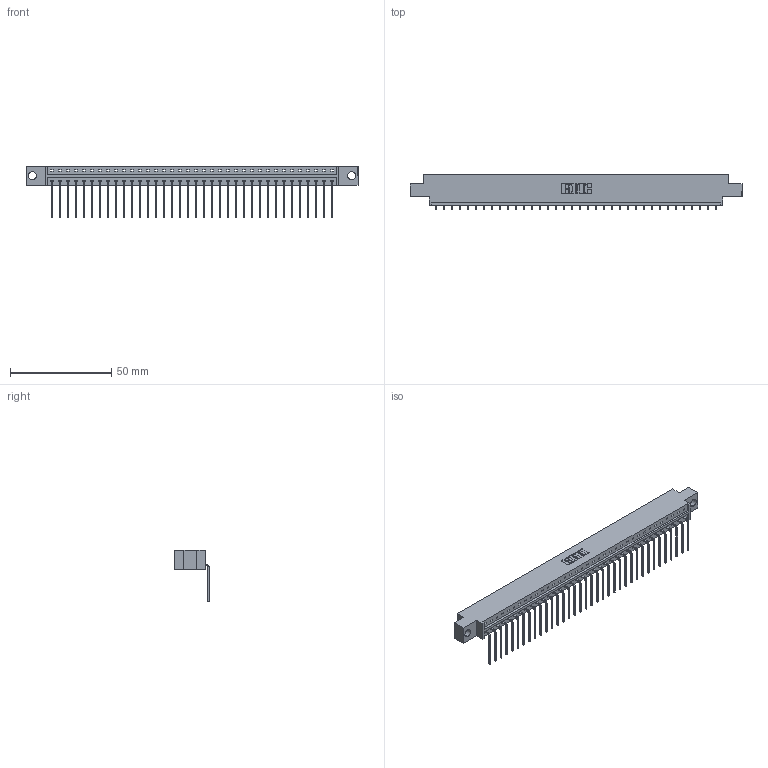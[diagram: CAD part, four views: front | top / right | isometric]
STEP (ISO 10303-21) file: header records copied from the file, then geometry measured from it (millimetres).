
FILE_DESCRIPTION (( 'STEP AP203' ), '1' );
FILE_NAME ('833-036-559-604.STEP', '2020-06-03T04:16:57', ( '' ), ( '' ), 'SwSTEP 2.0', 'SolidWorks 2020', '' );
FILE_SCHEMA (( 'CONFIG_CONTROL_DESIGN' ));
Length unit declared in the file: inch
Products named in the file (3): 345-292-001_558 559 Tail - 1; 833 Part_Offset - .156 Dia - TH; 833-036-559-604
Assembly tree (37 placements, depth 2):
  833-036-559-604
    833 Part_Offset - .156 Dia - TH
    345-292-001_558 559 Tail - 1  x36
Bounding box: 164.19 x 17.09 x 25.53 mm (x, y, z)
Volume: 16274.4 mm3; surface area: 18298.2 mm2
Topology: 37 solids, 37 shells, 2278 faces, 6875 edges, 4534 vertices
Faces by surface type: plane 1658, cylinder 620
Entity records: 23003 total; most frequent: CARTESIAN_POINT 3978, ORIENTED_EDGE 3950, DIRECTION 3367, EDGE_CURVE 1975, LINE 1847, VECTOR 1847, VERTEX_POINT 1314, AXIS2_PLACEMENT_3D 760
